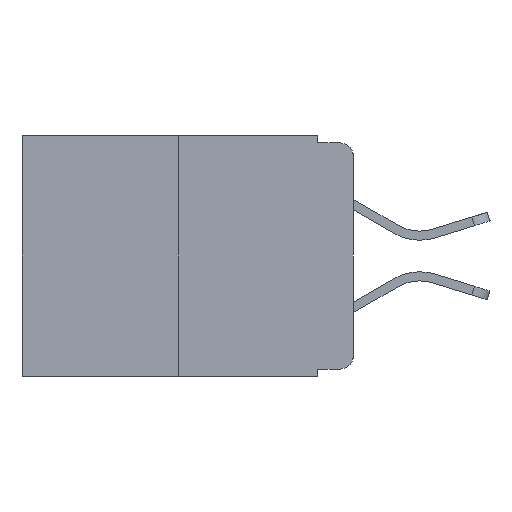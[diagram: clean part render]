
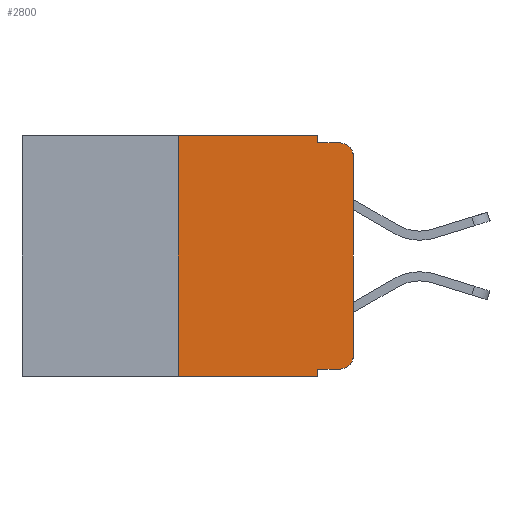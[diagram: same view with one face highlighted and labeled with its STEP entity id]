
A CAD part, left-side view. The second image highlights one B-rep face of the part: STEP entity #2800.
In plain terms, the highlighted planar face has unit normal (-1, 0, 0).
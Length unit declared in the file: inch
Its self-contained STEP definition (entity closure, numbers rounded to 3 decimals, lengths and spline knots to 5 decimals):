
#72 = DIRECTION ( 'NONE',  ( 0., -1., 0. ) ) ;
#350 = CIRCLE ( 'NONE', #13576, 0.02 ) ;
#526 = CARTESIAN_POINT ( 'NONE',  ( 0., 0.051, -0.01 ) ) ;
#648 = EDGE_CURVE ( 'NONE', #7624, #4613, #5977, .T. ) ;
#777 = DIRECTION ( 'NONE',  ( -1., 0., 0. ) ) ;
#1270 = EDGE_CURVE ( 'NONE', #9427, #14723, #18955, .T. ) ;
#1360 = VERTEX_POINT ( 'NONE', #13313 ) ;
#1636 = DIRECTION ( 'NONE',  ( 0., 0., 1. ) ) ;
#1722 = VERTEX_POINT ( 'NONE', #10166 ) ;
#2036 = EDGE_CURVE ( 'NONE', #17155, #9427, #350, .T. ) ;
#2125 = CARTESIAN_POINT ( 'NONE',  ( 0., 0.473, 0. ) ) ;
#2185 = ORIENTED_EDGE ( 'NONE', *, *, #9160, .F. ) ;
#2232 = CARTESIAN_POINT ( 'NONE',  ( 0., 0.051, 0. ) ) ;
#2381 = DIRECTION ( 'NONE',  ( -1., 0., 0. ) ) ;
#2682 = ORIENTED_EDGE ( 'NONE', *, *, #17684, .T. ) ;
#2800 = ADVANCED_FACE ( 'NONE', ( #18671 ), #8054, .F. ) ;
#2890 = CARTESIAN_POINT ( 'NONE',  ( 0., 0.051, 0. ) ) ;
#3795 = VECTOR ( 'NONE', #72, 39.37008 ) ;
#4613 = VERTEX_POINT ( 'NONE', #12476 ) ;
#4813 = AXIS2_PLACEMENT_3D ( 'NONE', #15767, #5444, #17217 ) ;
#5052 = LINE ( 'NONE', #2232, #10003 ) ;
#5415 = DIRECTION ( 'NONE',  ( 0., 0., -1. ) ) ;
#5444 = DIRECTION ( 'NONE',  ( 1., 0., 0. ) ) ;
#5564 = VECTOR ( 'NONE', #8887, 39.37008 ) ;
#5715 = EDGE_CURVE ( 'NONE', #7624, #14432, #13467, .T. ) ;
#5718 = CARTESIAN_POINT ( 'NONE',  ( 0., 0., 0. ) ) ;
#5873 = DIRECTION ( 'NONE',  ( 0., 0., -1. ) ) ;
#5977 = LINE ( 'NONE', #14847, #10247 ) ;
#6169 = DIRECTION ( 'NONE',  ( 0., -1., 0. ) ) ;
#7066 = CARTESIAN_POINT ( 'NONE',  ( 0., 0.051, -0.343 ) ) ;
#7624 = VERTEX_POINT ( 'NONE', #17961 ) ;
#8038 = LINE ( 'NONE', #2125, #11253 ) ;
#8054 = PLANE ( 'NONE',  #4813 ) ;
#8296 = CARTESIAN_POINT ( 'NONE',  ( 0., 0., -0.03 ) ) ;
#8887 = DIRECTION ( 'NONE',  ( 0., 0., 1. ) ) ;
#9063 = CARTESIAN_POINT ( 'NONE',  ( 0., 0., -0.313 ) ) ;
#9160 = EDGE_CURVE ( 'NONE', #1360, #14432, #5052, .T. ) ;
#9186 = EDGE_CURVE ( 'NONE', #4613, #1722, #8038, .T. ) ;
#9231 = ORIENTED_EDGE ( 'NONE', *, *, #13347, .T. ) ;
#9268 = EDGE_CURVE ( 'NONE', #1722, #18003, #15921, .T. ) ;
#9427 = VERTEX_POINT ( 'NONE', #9063 ) ;
#9520 = CARTESIAN_POINT ( 'NONE',  ( 0., 0.02, -0.01 ) ) ;
#10003 = VECTOR ( 'NONE', #10927, 39.37008 ) ;
#10166 = CARTESIAN_POINT ( 'NONE',  ( 0., 0.051, 0. ) ) ;
#10247 = VECTOR ( 'NONE', #1636, 39.37008 ) ;
#10790 = LINE ( 'NONE', #18339, #18930 ) ;
#10927 = DIRECTION ( 'NONE',  ( 0., 0., -1. ) ) ;
#11161 = ORIENTED_EDGE ( 'NONE', *, *, #12258, .F. ) ;
#11185 = ORIENTED_EDGE ( 'NONE', *, *, #5715, .T. ) ;
#11253 = VECTOR ( 'NONE', #17983, 39.37008 ) ;
#12080 = VERTEX_POINT ( 'NONE', #9520 ) ;
#12258 = EDGE_CURVE ( 'NONE', #18003, #12080, #17543, .T. ) ;
#12476 = CARTESIAN_POINT ( 'NONE',  ( 0., 0.25, 0. ) ) ;
#13078 = VECTOR ( 'NONE', #5873, 39.37008 ) ;
#13313 = CARTESIAN_POINT ( 'NONE',  ( 0., 0.051, -0.333 ) ) ;
#13347 = EDGE_CURVE ( 'NONE', #1360, #17155, #10790, .T. ) ;
#13467 = LINE ( 'NONE', #15220, #17884 ) ;
#13576 = AXIS2_PLACEMENT_3D ( 'NONE', #15612, #2381, #14142 ) ;
#14142 = DIRECTION ( 'NONE',  ( 0., 0., -1. ) ) ;
#14432 = VERTEX_POINT ( 'NONE', #7066 ) ;
#14551 = EDGE_LOOP ( 'NONE', ( #15535, #2682, #11161, #16731, #16714, #15528, #11185, #2185, #9231, #15210 ) ) ;
#14723 = VERTEX_POINT ( 'NONE', #8296 ) ;
#14847 = CARTESIAN_POINT ( 'NONE',  ( 0., 0.25, 0. ) ) ;
#15210 = ORIENTED_EDGE ( 'NONE', *, *, #2036, .T. ) ;
#15220 = CARTESIAN_POINT ( 'NONE',  ( 0., 0.473, -0.343 ) ) ;
#15317 = DIRECTION ( 'NONE',  ( 0., -1., 0. ) ) ;
#15528 = ORIENTED_EDGE ( 'NONE', *, *, #648, .F. ) ;
#15535 = ORIENTED_EDGE ( 'NONE', *, *, #1270, .T. ) ;
#15612 = CARTESIAN_POINT ( 'NONE',  ( 0., 0.02, -0.313 ) ) ;
#15767 = CARTESIAN_POINT ( 'NONE',  ( 0., 0.473, 0. ) ) ;
#15921 = LINE ( 'NONE', #2890, #13078 ) ;
#16196 = CARTESIAN_POINT ( 'NONE',  ( 0., 0.051, -0.01 ) ) ;
#16714 = ORIENTED_EDGE ( 'NONE', *, *, #9186, .F. ) ;
#16731 = ORIENTED_EDGE ( 'NONE', *, *, #9268, .F. ) ;
#16899 = CARTESIAN_POINT ( 'NONE',  ( 0., 0.02, -0.03 ) ) ;
#17155 = VERTEX_POINT ( 'NONE', #18278 ) ;
#17217 = DIRECTION ( 'NONE',  ( 0., 0., -1. ) ) ;
#17543 = LINE ( 'NONE', #16196, #3795 ) ;
#17587 = CIRCLE ( 'NONE', #17602, 0.02 ) ;
#17602 = AXIS2_PLACEMENT_3D ( 'NONE', #16899, #777, #5415 ) ;
#17684 = EDGE_CURVE ( 'NONE', #14723, #12080, #17587, .T. ) ;
#17884 = VECTOR ( 'NONE', #6169, 39.37008 ) ;
#17961 = CARTESIAN_POINT ( 'NONE',  ( 0., 0.25, -0.343 ) ) ;
#17983 = DIRECTION ( 'NONE',  ( 0., -1., 0. ) ) ;
#18003 = VERTEX_POINT ( 'NONE', #526 ) ;
#18278 = CARTESIAN_POINT ( 'NONE',  ( 0., 0.02, -0.333 ) ) ;
#18339 = CARTESIAN_POINT ( 'NONE',  ( 0., 0.051, -0.333 ) ) ;
#18671 = FACE_OUTER_BOUND ( 'NONE', #14551, .T. ) ;
#18930 = VECTOR ( 'NONE', #15317, 39.37008 ) ;
#18955 = LINE ( 'NONE', #5718, #5564 ) ;
